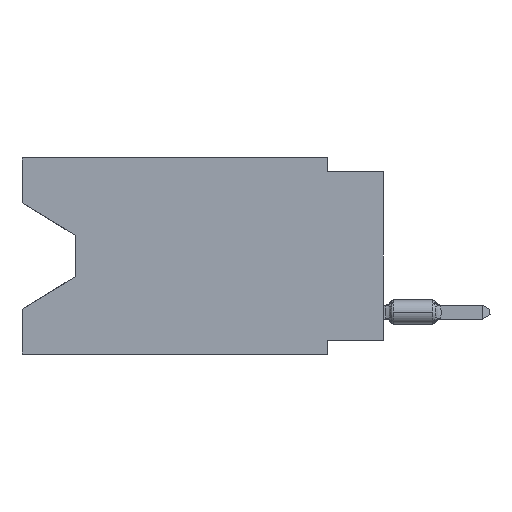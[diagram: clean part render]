
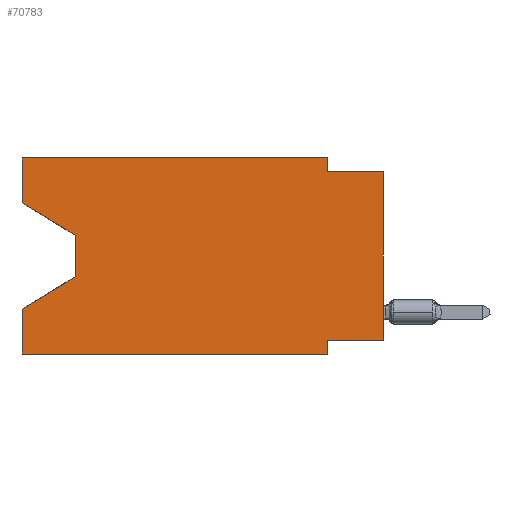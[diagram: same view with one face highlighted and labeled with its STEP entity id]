
A CAD part, left-side view. The second image highlights one B-rep face of the part: STEP entity #70783.
In plain terms, the highlighted planar face has unit normal (-1, 0, 0).
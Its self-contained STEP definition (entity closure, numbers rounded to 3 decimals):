
#730 = LINE ( 'NONE', #69872, #42992 ) ;
#1408 = VECTOR ( 'NONE', #41226, 1000. ) ;
#3241 = VECTOR ( 'NONE', #64187, 1000. ) ;
#3822 = VERTEX_POINT ( 'NONE', #70790 ) ;
#4052 = LINE ( 'NONE', #60856, #29274 ) ;
#4414 = VERTEX_POINT ( 'NONE', #71793 ) ;
#4592 = LINE ( 'NONE', #44924, #69109 ) ;
#5270 = CARTESIAN_POINT ( 'NONE',  ( 0., 2.54, -8.89 ) ) ;
#5551 = CARTESIAN_POINT ( 'NONE',  ( 0., 2.54, 0. ) ) ;
#5581 = FACE_OUTER_BOUND ( 'NONE', #13263, .T. ) ;
#5879 = CARTESIAN_POINT ( 'NONE',  ( 0., 2.54, -0.635 ) ) ;
#5943 = DIRECTION ( 'NONE',  ( 1., 0., 0. ) ) ;
#5952 = VERTEX_POINT ( 'NONE', #5879 ) ;
#6131 = LINE ( 'NONE', #17343, #1408 ) ;
#7237 = ORIENTED_EDGE ( 'NONE', *, *, #45271, .F. ) ;
#8298 = VERTEX_POINT ( 'NONE', #68219 ) ;
#8660 = VERTEX_POINT ( 'NONE', #10242 ) ;
#8682 = CARTESIAN_POINT ( 'NONE',  ( 0., 16.383, 0. ) ) ;
#8915 = ORIENTED_EDGE ( 'NONE', *, *, #51367, .T. ) ;
#9051 = DIRECTION ( 'NONE',  ( 0., -1., 0. ) ) ;
#9701 = EDGE_CURVE ( 'NONE', #41134, #53135, #11880, .T. ) ;
#9883 = LINE ( 'NONE', #67790, #12396 ) ;
#10242 = CARTESIAN_POINT ( 'NONE',  ( 0., 16.383, -6.852 ) ) ;
#11315 = DIRECTION ( 'NONE',  ( 0., 0., -1. ) ) ;
#11318 = EDGE_CURVE ( 'NONE', #3822, #25615, #37420, .T. ) ;
#11880 = LINE ( 'NONE', #57476, #3241 ) ;
#11898 = CARTESIAN_POINT ( 'NONE',  ( 0., 0., 0. ) ) ;
#12396 = VECTOR ( 'NONE', #55473, 1000. ) ;
#13263 = EDGE_LOOP ( 'NONE', ( #30895, #51901, #8915, #7237, #63449, #21774, #20838, #45258, #72214, #73828, #13653, #68631 ) ) ;
#13653 = ORIENTED_EDGE ( 'NONE', *, *, #11318, .F. ) ;
#16079 = VERTEX_POINT ( 'NONE', #28133 ) ;
#17163 = CARTESIAN_POINT ( 'NONE',  ( 0., 16.383, 0. ) ) ;
#17343 = CARTESIAN_POINT ( 'NONE',  ( 0., 16.383, 0. ) ) ;
#17565 = DIRECTION ( 'NONE',  ( 0., -0.855, -0.519 ) ) ;
#20494 = DIRECTION ( 'NONE',  ( 0., 0., -1. ) ) ;
#20838 = ORIENTED_EDGE ( 'NONE', *, *, #72547, .F. ) ;
#21774 = ORIENTED_EDGE ( 'NONE', *, *, #31132, .F. ) ;
#22118 = EDGE_CURVE ( 'NONE', #25713, #4414, #730, .T. ) ;
#22229 = VECTOR ( 'NONE', #39383, 1000. ) ;
#25615 = VERTEX_POINT ( 'NONE', #5551 ) ;
#25713 = VERTEX_POINT ( 'NONE', #72343 ) ;
#27970 = VERTEX_POINT ( 'NONE', #73351 ) ;
#28133 = CARTESIAN_POINT ( 'NONE',  ( 0., 0., -0.635 ) ) ;
#28770 = AXIS2_PLACEMENT_3D ( 'NONE', #17163, #5943, #51529 ) ;
#28842 = EDGE_CURVE ( 'NONE', #4414, #38397, #4052, .T. ) ;
#29274 = VECTOR ( 'NONE', #20494, 1000. ) ;
#29497 = CARTESIAN_POINT ( 'NONE',  ( 0., 2.54, 0. ) ) ;
#30708 = CARTESIAN_POINT ( 'NONE',  ( 0., 16.383, -8.89 ) ) ;
#30895 = ORIENTED_EDGE ( 'NONE', *, *, #22118, .T. ) ;
#31132 = EDGE_CURVE ( 'NONE', #8298, #53135, #62207, .T. ) ;
#32805 = EDGE_CURVE ( 'NONE', #5952, #16079, #4592, .T. ) ;
#33206 = LINE ( 'NONE', #11898, #36682 ) ;
#36682 = VECTOR ( 'NONE', #45157, 1000. ) ;
#36955 = EDGE_CURVE ( 'NONE', #25615, #5952, #62138, .T. ) ;
#37420 = LINE ( 'NONE', #8682, #42840 ) ;
#38397 = VERTEX_POINT ( 'NONE', #39570 ) ;
#39383 = DIRECTION ( 'NONE',  ( 0., 0., -1. ) ) ;
#39570 = CARTESIAN_POINT ( 'NONE',  ( 0., 13.97, -5.385 ) ) ;
#41134 = VERTEX_POINT ( 'NONE', #30708 ) ;
#41226 = DIRECTION ( 'NONE',  ( 0., 0., 1. ) ) ;
#42840 = VECTOR ( 'NONE', #9051, 1000. ) ;
#42992 = VECTOR ( 'NONE', #17565, 1000. ) ;
#44924 = CARTESIAN_POINT ( 'NONE',  ( 0., 0., -0.635 ) ) ;
#45157 = DIRECTION ( 'NONE',  ( 0., 0., 1. ) ) ;
#45258 = ORIENTED_EDGE ( 'NONE', *, *, #54947, .T. ) ;
#45271 = EDGE_CURVE ( 'NONE', #41134, #8660, #63139, .T. ) ;
#46442 = DIRECTION ( 'NONE',  ( 0., 0.855, -0.519 ) ) ;
#47413 = EDGE_CURVE ( 'NONE', #25713, #3822, #6131, .T. ) ;
#48464 = VECTOR ( 'NONE', #72872, 1000. ) ;
#51367 = EDGE_CURVE ( 'NONE', #38397, #8660, #58430, .T. ) ;
#51529 = DIRECTION ( 'NONE',  ( 0., 0., -1. ) ) ;
#51901 = ORIENTED_EDGE ( 'NONE', *, *, #28842, .T. ) ;
#52272 = PLANE ( 'NONE',  #28770 ) ;
#53135 = VERTEX_POINT ( 'NONE', #5270 ) ;
#54947 = EDGE_CURVE ( 'NONE', #27970, #16079, #33206, .T. ) ;
#55473 = DIRECTION ( 'NONE',  ( 0., 1., 0. ) ) ;
#57476 = CARTESIAN_POINT ( 'NONE',  ( 0., 16.383, -8.89 ) ) ;
#58066 = CARTESIAN_POINT ( 'NONE',  ( 0., 13.97, -5.385 ) ) ;
#58430 = LINE ( 'NONE', #58066, #68506 ) ;
#60856 = CARTESIAN_POINT ( 'NONE',  ( 0., 13.97, -3.505 ) ) ;
#61666 = CARTESIAN_POINT ( 'NONE',  ( 0., 16.383, 0. ) ) ;
#62138 = LINE ( 'NONE', #29497, #63244 ) ;
#62207 = LINE ( 'NONE', #67820, #22229 ) ;
#63139 = LINE ( 'NONE', #61666, #48464 ) ;
#63244 = VECTOR ( 'NONE', #11315, 1000. ) ;
#63449 = ORIENTED_EDGE ( 'NONE', *, *, #9701, .T. ) ;
#64187 = DIRECTION ( 'NONE',  ( 0., -1., 0. ) ) ;
#67790 = CARTESIAN_POINT ( 'NONE',  ( 0., 0., -8.255 ) ) ;
#67820 = CARTESIAN_POINT ( 'NONE',  ( 0., 2.54, -8.89 ) ) ;
#68219 = CARTESIAN_POINT ( 'NONE',  ( 0., 2.54, -8.255 ) ) ;
#68506 = VECTOR ( 'NONE', #46442, 1000. ) ;
#68631 = ORIENTED_EDGE ( 'NONE', *, *, #47413, .F. ) ;
#69109 = VECTOR ( 'NONE', #72613, 1000. ) ;
#69872 = CARTESIAN_POINT ( 'NONE',  ( 0., 16.383, -2.038 ) ) ;
#70783 = ADVANCED_FACE ( 'NONE', ( #5581 ), #52272, .F. ) ;
#70790 = CARTESIAN_POINT ( 'NONE',  ( 0., 16.383, 0. ) ) ;
#71793 = CARTESIAN_POINT ( 'NONE',  ( 0., 13.97, -3.505 ) ) ;
#72214 = ORIENTED_EDGE ( 'NONE', *, *, #32805, .F. ) ;
#72343 = CARTESIAN_POINT ( 'NONE',  ( 0., 16.383, -2.038 ) ) ;
#72547 = EDGE_CURVE ( 'NONE', #27970, #8298, #9883, .T. ) ;
#72613 = DIRECTION ( 'NONE',  ( 0., -1., 0. ) ) ;
#72872 = DIRECTION ( 'NONE',  ( 0., 0., 1. ) ) ;
#73351 = CARTESIAN_POINT ( 'NONE',  ( 0., 0., -8.255 ) ) ;
#73828 = ORIENTED_EDGE ( 'NONE', *, *, #36955, .F. ) ;
